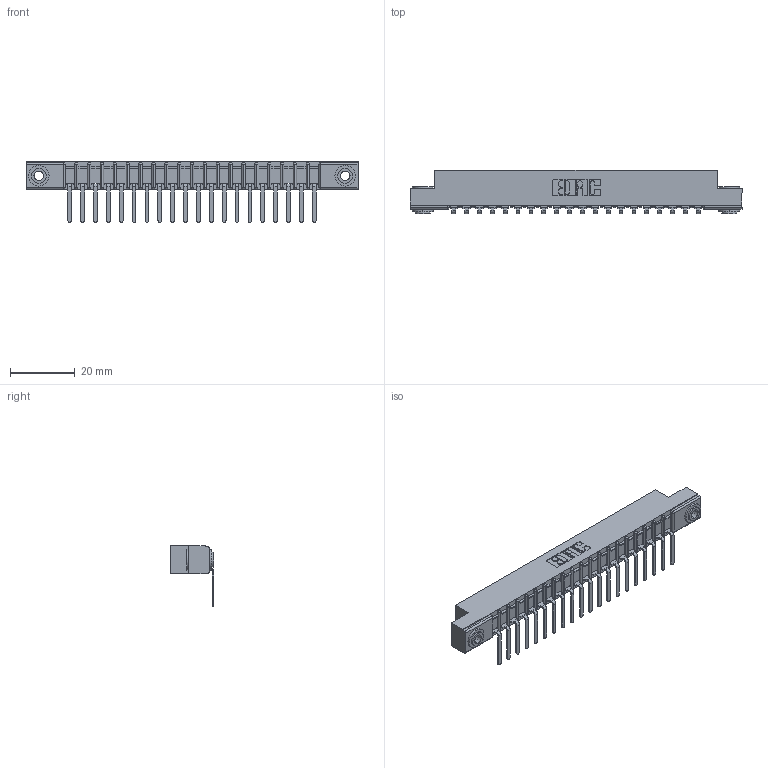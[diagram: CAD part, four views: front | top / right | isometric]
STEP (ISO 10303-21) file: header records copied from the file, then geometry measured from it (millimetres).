
FILE_DESCRIPTION (( 'STEP AP203' ), '1' );
FILE_NAME ('307-020-557-103.STEP', '2019-09-04T23:19:03', ( '' ), ( '' ), 'SwSTEP 2.0', 'SolidWorks 2016', '' );
FILE_SCHEMA (( 'CONFIG_CONTROL_DESIGN' ));
Length unit declared in the file: inch
Products named in the file (4): 307 Part_.156 Dia Mounting Holes; 307-020-557-103; 307-290-002_557; 345-250-002_345-250-002-102
Assembly tree (23 placements, depth 2):
  307-020-557-103
    307 Part_.156 Dia Mounting Holes
    307-290-002_557  x20
    345-250-002_345-250-002-102  x2
Bounding box: 102.26 x 13.36 x 18.67 mm (x, y, z)
Volume: 6805.3 mm3; surface area: 12840.2 mm2
Topology: 23 solids, 23 shells, 1751 faces, 5315 edges, 3482 vertices
Faces by surface type: plane 1034, cylinder 667, sphere 42, cone 8
Entity records: 21777 total; most frequent: CARTESIAN_POINT 3649, ORIENTED_EDGE 3630, DIRECTION 3571, EDGE_CURVE 1815, LINE 1371, VECTOR 1371, VERTEX_POINT 1178, AXIS2_PLACEMENT_3D 1100
